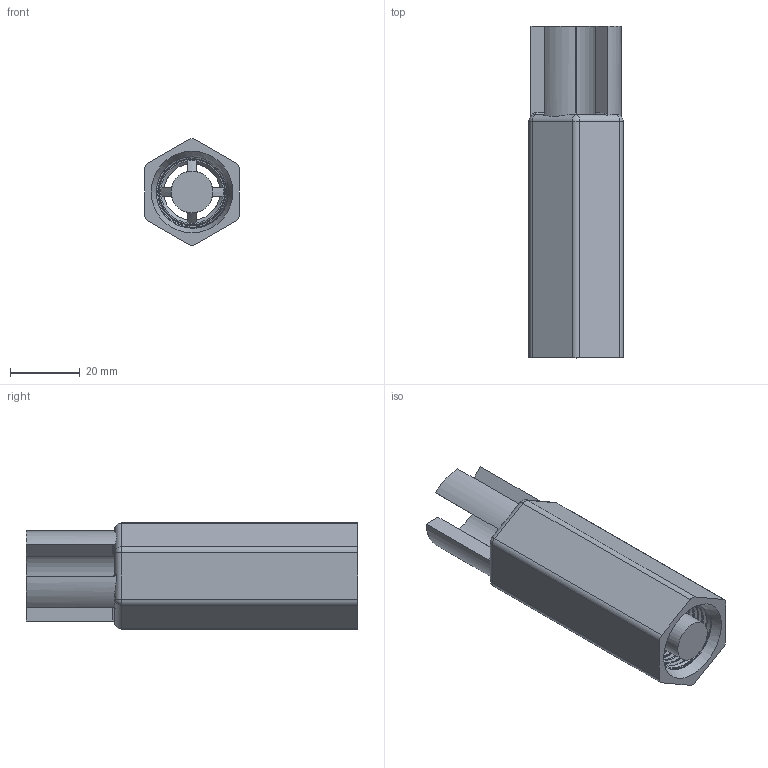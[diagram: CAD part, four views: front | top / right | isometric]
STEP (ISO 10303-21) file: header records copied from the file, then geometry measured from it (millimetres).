
FILE_DESCRIPTION(/* description */ (''),/* implementation_level */ '2;1');
FILE_NAME(/* name */ 'Fitting Metric (6mm).stp',/* time_stamp */ '2021-02-15T01:40:59-06:00',/* author */ ('johne'),/* organization */ (''),/* preprocessor_version */ 'ST-DEVELOPER v18',/* originating_system */ 'Autodesk Inventor 2020',/* authorisation */ '');
FILE_SCHEMA (('AUTOMOTIVE_DESIGN { 1 0 10303 214 3 1 1 }'));
Length unit declared in the file: inch
Products named in the file (1): Fitting for 6mm Rod V2
Bounding box: 27.05 x 95.25 x 30.61 mm (x, y, z)
Volume: 33481.6 mm3; surface area: 17175.3 mm2
Topology: 1 solids, 1 shells, 127 faces, 369 edges, 240 vertices
Faces by surface type: cylinder 52, plane 42, cone 10, bspline 10, torus 7, sphere 6
Full cylindrical faces by diameter (mm): 6.3 x1, 9.052 x1, 12 x1, 16.2 x1, 20.955 x12
Entity records: 13287 total; most frequent: CARTESIAN_POINT 10070, ORIENTED_EDGE 738, DIRECTION 587, EDGE_CURVE 369, VERTEX_POINT 240, AXIS2_PLACEMENT_3D 229, EDGE_LOOP 131, LINE 129
